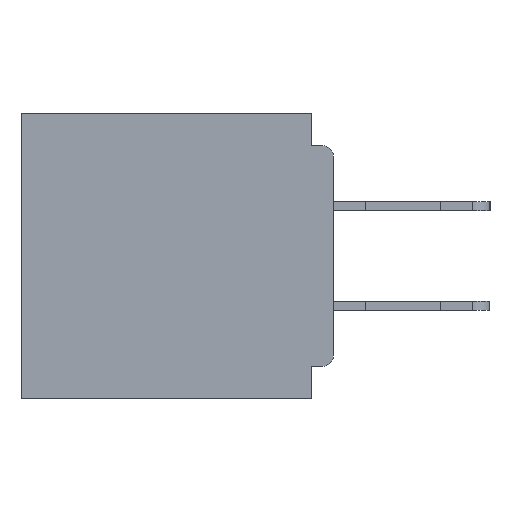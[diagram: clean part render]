
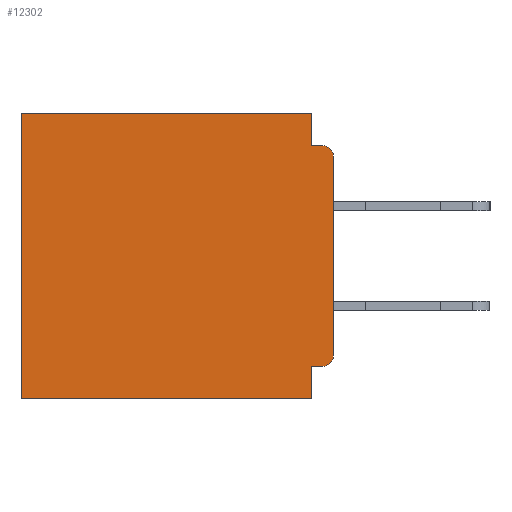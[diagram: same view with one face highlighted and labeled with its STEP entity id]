
A CAD part, left-side view. The second image highlights one B-rep face of the part: STEP entity #12302.
In plain terms, the highlighted planar face has unit normal (-1, 0, 0).
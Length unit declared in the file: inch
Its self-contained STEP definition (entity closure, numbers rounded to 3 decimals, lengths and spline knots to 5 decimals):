
#1705 = EDGE_CURVE ( 'NONE', #10308, #25641, #44031, .T. ) ;
#3371 = AXIS2_PLACEMENT_3D ( 'NONE', #17013, #42575, #20732 ) ;
#3570 = EDGE_CURVE ( 'NONE', #44790, #11787, #32504, .T. ) ;
#3836 = ORIENTED_EDGE ( 'NONE', *, *, #17003, .F. ) ;
#3930 = PLANE ( 'NONE',  #22501 ) ;
#4553 = CARTESIAN_POINT ( 'NONE',  ( 0.3, 0.031, -0.045 ) ) ;
#4957 = CARTESIAN_POINT ( 'NONE',  ( 0.3, 0.437, -0.4 ) ) ;
#5568 = CARTESIAN_POINT ( 'NONE',  ( 0.3, 0.031, -0.355 ) ) ;
#6088 = VERTEX_POINT ( 'NONE', #4957 ) ;
#6250 = LINE ( 'NONE', #23244, #23410 ) ;
#6727 = ORIENTED_EDGE ( 'NONE', *, *, #18721, .T. ) ;
#7576 = DIRECTION ( 'NONE',  ( 1., 0., 0. ) ) ;
#7727 = ORIENTED_EDGE ( 'NONE', *, *, #3570, .T. ) ;
#7832 = VECTOR ( 'NONE', #46903, 39.37008 ) ;
#8003 = VERTEX_POINT ( 'NONE', #5568 ) ;
#8656 = DIRECTION ( 'NONE',  ( 0., 0., -1. ) ) ;
#8865 = ORIENTED_EDGE ( 'NONE', *, *, #40093, .F. ) ;
#9236 = CARTESIAN_POINT ( 'NONE',  ( 0.3, 0., -0.4 ) ) ;
#9450 = VECTOR ( 'NONE', #35030, 39.37008 ) ;
#10308 = VERTEX_POINT ( 'NONE', #33862 ) ;
#11787 = VERTEX_POINT ( 'NONE', #44131 ) ;
#12292 = EDGE_LOOP ( 'NONE', ( #19904, #34771, #16031, #39771, #7727, #39267, #12795, #3836, #8865, #6727 ) ) ;
#12302 = ADVANCED_FACE ( 'NONE', ( #21385 ), #3930, .F. ) ;
#12795 = ORIENTED_EDGE ( 'NONE', *, *, #12963, .F. ) ;
#12842 = CARTESIAN_POINT ( 'NONE',  ( 0.3, 0.015, -0.355 ) ) ;
#12963 = EDGE_CURVE ( 'NONE', #45885, #6088, #40119, .T. ) ;
#13067 = VECTOR ( 'NONE', #27144, 39.37008 ) ;
#13140 = VECTOR ( 'NONE', #20287, 39.37008 ) ;
#13544 = DIRECTION ( 'NONE',  ( 0., 0., -1. ) ) ;
#14469 = CARTESIAN_POINT ( 'NONE',  ( 0.3, 0.015, -0.06 ) ) ;
#14568 = VECTOR ( 'NONE', #13544, 39.37008 ) ;
#14922 = EDGE_CURVE ( 'NONE', #10308, #34881, #25188, .T. ) ;
#16031 = ORIENTED_EDGE ( 'NONE', *, *, #43529, .F. ) ;
#17003 = EDGE_CURVE ( 'NONE', #8003, #45885, #18668, .T. ) ;
#17013 = CARTESIAN_POINT ( 'NONE',  ( 0.3, 0.015, -0.34 ) ) ;
#17293 = CARTESIAN_POINT ( 'NONE',  ( 0.3, 0., 0. ) ) ;
#18094 = DIRECTION ( 'NONE',  ( -1., 0., 0. ) ) ;
#18513 = CARTESIAN_POINT ( 'NONE',  ( 0.3, 0., -0.4 ) ) ;
#18668 = LINE ( 'NONE', #21420, #7832 ) ;
#18721 = EDGE_CURVE ( 'NONE', #37820, #34881, #34192, .T. ) ;
#19556 = CARTESIAN_POINT ( 'NONE',  ( 0.3, 0.031, -0.4 ) ) ;
#19904 = ORIENTED_EDGE ( 'NONE', *, *, #14922, .F. ) ;
#20287 = DIRECTION ( 'NONE',  ( 0., 0., -1. ) ) ;
#20357 = LINE ( 'NONE', #42395, #9450 ) ;
#20732 = DIRECTION ( 'NONE',  ( 0., 0., -1. ) ) ;
#20739 = VECTOR ( 'NONE', #36720, 39.37008 ) ;
#20779 = CARTESIAN_POINT ( 'NONE',  ( 0.3, 0.031, 0. ) ) ;
#21084 = CARTESIAN_POINT ( 'NONE',  ( 0.3, 0.015, -0.045 ) ) ;
#21385 = FACE_OUTER_BOUND ( 'NONE', #12292, .T. ) ;
#21420 = CARTESIAN_POINT ( 'NONE',  ( 0.3, 0.031, -0.4 ) ) ;
#22501 = AXIS2_PLACEMENT_3D ( 'NONE', #43926, #7576, #33086 ) ;
#23244 = CARTESIAN_POINT ( 'NONE',  ( 0.3, 0., -0.355 ) ) ;
#23410 = VECTOR ( 'NONE', #41537, 39.37008 ) ;
#24433 = CARTESIAN_POINT ( 'NONE',  ( 0.3, 0.031, 0. ) ) ;
#24533 = LINE ( 'NONE', #30393, #42789 ) ;
#25188 = LINE ( 'NONE', #9236, #13140 ) ;
#25641 = VERTEX_POINT ( 'NONE', #21084 ) ;
#27144 = DIRECTION ( 'NONE',  ( 0., 1., 0. ) ) ;
#27608 = DIRECTION ( 'NONE',  ( 0., 0., -1. ) ) ;
#30393 = CARTESIAN_POINT ( 'NONE',  ( 0.3, 0.437, -0.4 ) ) ;
#32504 = LINE ( 'NONE', #17293, #13067 ) ;
#33086 = DIRECTION ( 'NONE',  ( 0., 0., -1. ) ) ;
#33862 = CARTESIAN_POINT ( 'NONE',  ( 0.3, 0., -0.06 ) ) ;
#33983 = LINE ( 'NONE', #20779, #14568 ) ;
#34192 = CIRCLE ( 'NONE', #3371, 0.015 ) ;
#34771 = ORIENTED_EDGE ( 'NONE', *, *, #1705, .T. ) ;
#34881 = VERTEX_POINT ( 'NONE', #46014 ) ;
#35030 = DIRECTION ( 'NONE',  ( 0., -1., 0. ) ) ;
#36720 = DIRECTION ( 'NONE',  ( 0., 1., 0. ) ) ;
#37820 = VERTEX_POINT ( 'NONE', #12842 ) ;
#39267 = ORIENTED_EDGE ( 'NONE', *, *, #40088, .T. ) ;
#39771 = ORIENTED_EDGE ( 'NONE', *, *, #44791, .F. ) ;
#39820 = AXIS2_PLACEMENT_3D ( 'NONE', #14469, #18094, #27608 ) ;
#39991 = VERTEX_POINT ( 'NONE', #4553 ) ;
#40088 = EDGE_CURVE ( 'NONE', #11787, #6088, #24533, .T. ) ;
#40093 = EDGE_CURVE ( 'NONE', #37820, #8003, #6250, .T. ) ;
#40119 = LINE ( 'NONE', #18513, #20739 ) ;
#41537 = DIRECTION ( 'NONE',  ( 0., 1., 0. ) ) ;
#42395 = CARTESIAN_POINT ( 'NONE',  ( 0.3, 0., -0.045 ) ) ;
#42575 = DIRECTION ( 'NONE',  ( -1., 0., 0. ) ) ;
#42789 = VECTOR ( 'NONE', #8656, 39.37008 ) ;
#43529 = EDGE_CURVE ( 'NONE', #39991, #25641, #20357, .T. ) ;
#43926 = CARTESIAN_POINT ( 'NONE',  ( 0.3, 0., -0.4 ) ) ;
#44031 = CIRCLE ( 'NONE', #39820, 0.015 ) ;
#44131 = CARTESIAN_POINT ( 'NONE',  ( 0.3, 0.437, 0. ) ) ;
#44790 = VERTEX_POINT ( 'NONE', #24433 ) ;
#44791 = EDGE_CURVE ( 'NONE', #44790, #39991, #33983, .T. ) ;
#45885 = VERTEX_POINT ( 'NONE', #19556 ) ;
#46014 = CARTESIAN_POINT ( 'NONE',  ( 0.3, 0., -0.34 ) ) ;
#46903 = DIRECTION ( 'NONE',  ( 0., 0., -1. ) ) ;
